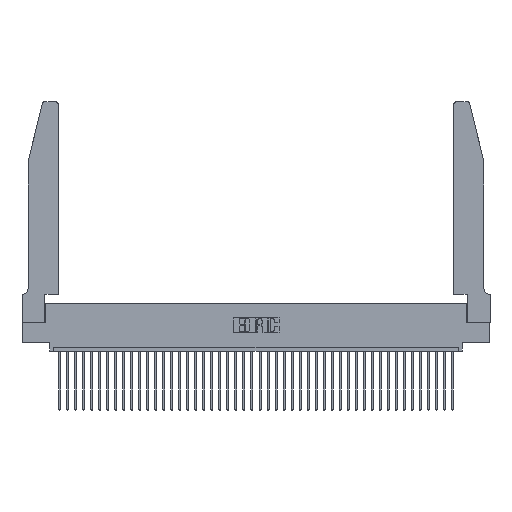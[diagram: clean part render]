
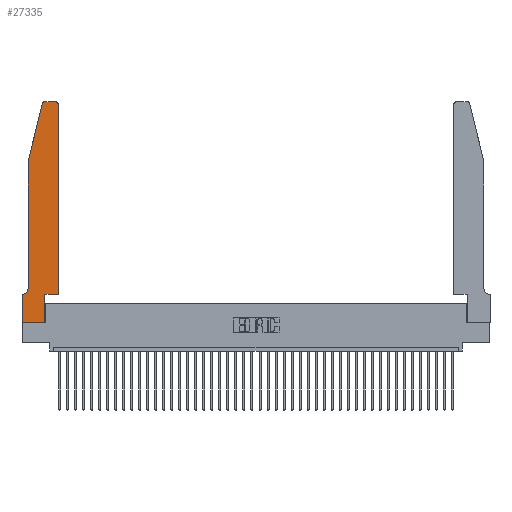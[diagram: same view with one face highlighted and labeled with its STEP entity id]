
A CAD part, top view. The second image highlights one B-rep face of the part: STEP entity #27335.
In plain terms, the highlighted planar face has unit normal (0, 0, 1).
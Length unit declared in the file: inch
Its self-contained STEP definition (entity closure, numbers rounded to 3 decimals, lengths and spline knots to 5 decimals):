
#383 = ORIENTED_EDGE ( 'NONE', *, *, #28475, .T. ) ;
#554 = CARTESIAN_POINT ( 'NONE',  ( 0.284, 2.75, 0.37 ) ) ;
#1500 = VECTOR ( 'NONE', #17679, 39.37008 ) ;
#2561 = DIRECTION ( 'NONE',  ( 1., 0., 0. ) ) ;
#3320 = CARTESIAN_POINT ( 'NONE',  ( 0., 0., 0.37 ) ) ;
#4015 = CARTESIAN_POINT ( 'NONE',  ( 0., 0., 0.37 ) ) ;
#4068 = DIRECTION ( 'NONE',  ( 1., 0., 0. ) ) ;
#4265 = CIRCLE ( 'NONE', #35732, 0.03 ) ;
#4296 = CARTESIAN_POINT ( 'NONE',  ( 0.2865, 0.35, 0.37 ) ) ;
#4352 = CARTESIAN_POINT ( 'NONE',  ( 0.2605, 2.75, 0.37 ) ) ;
#5255 = CARTESIAN_POINT ( 'NONE',  ( 0., 0., 0.37 ) ) ;
#6119 = ORIENTED_EDGE ( 'NONE', *, *, #38800, .T. ) ;
#6215 = CIRCLE ( 'NONE', #16678, 0.07 ) ;
#6489 = VERTEX_POINT ( 'NONE', #15505 ) ;
#6694 = ORIENTED_EDGE ( 'NONE', *, *, #23056, .T. ) ;
#7159 = EDGE_CURVE ( 'NONE', #29307, #37474, #17086, .T. ) ;
#7573 = VECTOR ( 'NONE', #15103, 39.37008 ) ;
#7933 = VECTOR ( 'NONE', #32794, 39.37008 ) ;
#8803 = VERTEX_POINT ( 'NONE', #36408 ) ;
#10089 = EDGE_CURVE ( 'NONE', #19683, #8803, #4265, .T. ) ;
#10630 = DIRECTION ( 'NONE',  ( 1., 0., 0. ) ) ;
#10736 = CARTESIAN_POINT ( 'NONE',  ( 0.2865, 0.35, 0.37 ) ) ;
#12549 = EDGE_LOOP ( 'NONE', ( #6119, #6694, #30839, #41184, #35921, #33345, #26222, #383, #40614, #29750, #29318, #38863 ) ) ;
#12685 = FACE_OUTER_BOUND ( 'NONE', #12549, .T. ) ;
#12852 = VERTEX_POINT ( 'NONE', #30139 ) ;
#12940 = LINE ( 'NONE', #4352, #38518 ) ;
#13269 = CARTESIAN_POINT ( 'NONE',  ( 0.0055, 0.42, 0.37 ) ) ;
#15034 = LINE ( 'NONE', #36856, #1500 ) ;
#15103 = DIRECTION ( 'NONE',  ( -1., 0., 0. ) ) ;
#15505 = CARTESIAN_POINT ( 'NONE',  ( 0.4505, 0.35, 0.37 ) ) ;
#15579 = CARTESIAN_POINT ( 'NONE',  ( 0.0755, 2., 0.37 ) ) ;
#16678 = AXIS2_PLACEMENT_3D ( 'NONE', #13269, #22465, #32459 ) ;
#16923 = PLANE ( 'NONE',  #39995 ) ;
#17086 = LINE ( 'NONE', #37388, #7573 ) ;
#17232 = DIRECTION ( 'NONE',  ( -1., 0., 0. ) ) ;
#17679 = DIRECTION ( 'NONE',  ( 1., 0., 0. ) ) ;
#17867 = DIRECTION ( 'NONE',  ( 1., 0., 0. ) ) ;
#17998 = LINE ( 'NONE', #24362, #26943 ) ;
#18675 = CARTESIAN_POINT ( 'NONE',  ( 0.25487, 2.72718, 0.37 ) ) ;
#18952 = VERTEX_POINT ( 'NONE', #554 ) ;
#19356 = CARTESIAN_POINT ( 'NONE',  ( 0., 0.35, 0.37 ) ) ;
#19683 = VERTEX_POINT ( 'NONE', #30672 ) ;
#19740 = CIRCLE ( 'NONE', #29626, 0.03 ) ;
#19855 = VECTOR ( 'NONE', #23640, 39.37008 ) ;
#21104 = VERTEX_POINT ( 'NONE', #4015 ) ;
#21292 = EDGE_CURVE ( 'NONE', #6489, #19683, #17998, .T. ) ;
#21375 = EDGE_CURVE ( 'NONE', #22720, #29346, #34503, .T. ) ;
#21482 = CARTESIAN_POINT ( 'NONE',  ( 0.284, 2.72, 0.37 ) ) ;
#22053 = DIRECTION ( 'NONE',  ( 0., -1., 0. ) ) ;
#22095 = EDGE_CURVE ( 'NONE', #25456, #22111, #29367, .T. ) ;
#22111 = VERTEX_POINT ( 'NONE', #4296 ) ;
#22212 = VECTOR ( 'NONE', #17867, 39.37008 ) ;
#22465 = DIRECTION ( 'NONE',  ( 0., 0., -1. ) ) ;
#22720 = VERTEX_POINT ( 'NONE', #18675 ) ;
#23056 = EDGE_CURVE ( 'NONE', #18952, #22720, #19740, .T. ) ;
#23133 = LINE ( 'NONE', #5255, #22212 ) ;
#23300 = CARTESIAN_POINT ( 'NONE',  ( 0.0755, 2., 0.37 ) ) ;
#23640 = DIRECTION ( 'NONE',  ( 0., 1., 0. ) ) ;
#23676 = CARTESIAN_POINT ( 'NONE',  ( 0., 0.35, 0.37 ) ) ;
#24189 = VECTOR ( 'NONE', #35000, 39.37008 ) ;
#24362 = CARTESIAN_POINT ( 'NONE',  ( 0.4505, 0.35, 0.37 ) ) ;
#25091 = VECTOR ( 'NONE', #22053, 39.37008 ) ;
#25341 = CARTESIAN_POINT ( 'NONE',  ( 0.0055, 0.35, 0.37 ) ) ;
#25456 = VERTEX_POINT ( 'NONE', #39806 ) ;
#26222 = ORIENTED_EDGE ( 'NONE', *, *, #35003, .T. ) ;
#26865 = DIRECTION ( 'NONE',  ( 0., 0., 1. ) ) ;
#26943 = VECTOR ( 'NONE', #40596, 39.37008 ) ;
#27335 = ADVANCED_FACE ( 'NONE', ( #12685 ), #16923, .T. ) ;
#28475 = EDGE_CURVE ( 'NONE', #21104, #25456, #23133, .T. ) ;
#29307 = VERTEX_POINT ( 'NONE', #25341 ) ;
#29318 = ORIENTED_EDGE ( 'NONE', *, *, #21292, .T. ) ;
#29346 = VERTEX_POINT ( 'NONE', #29601 ) ;
#29367 = LINE ( 'NONE', #10736, #19855 ) ;
#29601 = CARTESIAN_POINT ( 'NONE',  ( 0.0755, 2., 0.37 ) ) ;
#29626 = AXIS2_PLACEMENT_3D ( 'NONE', #21482, #37429, #2561 ) ;
#29672 = CARTESIAN_POINT ( 'NONE',  ( 0.4205, 2.72, 0.37 ) ) ;
#29750 = ORIENTED_EDGE ( 'NONE', *, *, #37780, .T. ) ;
#30139 = CARTESIAN_POINT ( 'NONE',  ( 0.0755, 0.42, 0.37 ) ) ;
#30672 = CARTESIAN_POINT ( 'NONE',  ( 0.4505, 2.72, 0.37 ) ) ;
#30839 = ORIENTED_EDGE ( 'NONE', *, *, #21375, .T. ) ;
#32459 = DIRECTION ( 'NONE',  ( -1., 0., 0. ) ) ;
#32625 = LINE ( 'NONE', #3320, #24189 ) ;
#32794 = DIRECTION ( 'NONE',  ( -0.239, -0.971, 0. ) ) ;
#33345 = ORIENTED_EDGE ( 'NONE', *, *, #7159, .T. ) ;
#34503 = LINE ( 'NONE', #23300, #7933 ) ;
#35000 = DIRECTION ( 'NONE',  ( 0., -1., 0. ) ) ;
#35003 = EDGE_CURVE ( 'NONE', #37474, #21104, #32625, .T. ) ;
#35732 = AXIS2_PLACEMENT_3D ( 'NONE', #29672, #39786, #4068 ) ;
#35921 = ORIENTED_EDGE ( 'NONE', *, *, #37463, .T. ) ;
#36136 = EDGE_CURVE ( 'NONE', #29346, #12852, #39022, .T. ) ;
#36408 = CARTESIAN_POINT ( 'NONE',  ( 0.4205, 2.75, 0.37 ) ) ;
#36856 = CARTESIAN_POINT ( 'NONE',  ( 0.4505, 0.35, 0.37 ) ) ;
#37388 = CARTESIAN_POINT ( 'NONE',  ( 0.0755, 0.35, 0.37 ) ) ;
#37429 = DIRECTION ( 'NONE',  ( 0., 0., 1. ) ) ;
#37463 = EDGE_CURVE ( 'NONE', #12852, #29307, #6215, .T. ) ;
#37474 = VERTEX_POINT ( 'NONE', #19356 ) ;
#37780 = EDGE_CURVE ( 'NONE', #22111, #6489, #15034, .T. ) ;
#38518 = VECTOR ( 'NONE', #17232, 39.37008 ) ;
#38800 = EDGE_CURVE ( 'NONE', #8803, #18952, #12940, .T. ) ;
#38863 = ORIENTED_EDGE ( 'NONE', *, *, #10089, .T. ) ;
#39022 = LINE ( 'NONE', #15579, #25091 ) ;
#39786 = DIRECTION ( 'NONE',  ( 0., 0., 1. ) ) ;
#39806 = CARTESIAN_POINT ( 'NONE',  ( 0.2865, 0., 0.37 ) ) ;
#39995 = AXIS2_PLACEMENT_3D ( 'NONE', #23676, #26865, #10630 ) ;
#40596 = DIRECTION ( 'NONE',  ( 0., 1., 0. ) ) ;
#40614 = ORIENTED_EDGE ( 'NONE', *, *, #22095, .T. ) ;
#41184 = ORIENTED_EDGE ( 'NONE', *, *, #36136, .T. ) ;
